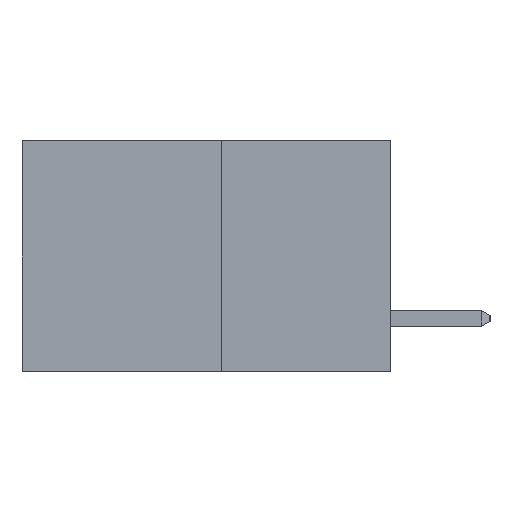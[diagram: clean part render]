
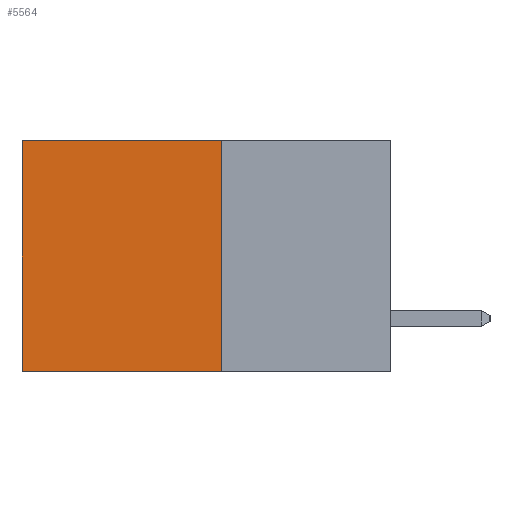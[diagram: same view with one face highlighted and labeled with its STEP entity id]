
A CAD part, left-side view. The second image highlights one B-rep face of the part: STEP entity #5564.
In plain terms, the highlighted planar face has unit normal (-1, 0, 0).
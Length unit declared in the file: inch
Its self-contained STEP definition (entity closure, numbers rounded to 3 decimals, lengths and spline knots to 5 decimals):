
#116 = VERTEX_POINT ( 'NONE', #3223 ) ;
#127 = EDGE_CURVE ( 'NONE', #1532, #116, #7901, .T. ) ;
#175 = ORIENTED_EDGE ( 'NONE', *, *, #199, .T. ) ;
#199 = EDGE_CURVE ( 'NONE', #2654, #116, #7151, .T. ) ;
#217 = VECTOR ( 'NONE', #4438, 39.37008 ) ;
#226 = ORIENTED_EDGE ( 'NONE', *, *, #127, .F. ) ;
#299 = DIRECTION ( 'NONE',  ( 0., 1., 0. ) ) ;
#313 = ORIENTED_EDGE ( 'NONE', *, *, #3070, .F. ) ;
#405 = ORIENTED_EDGE ( 'NONE', *, *, #1377, .T. ) ;
#804 = DIRECTION ( 'NONE',  ( 0., 1., 0. ) ) ;
#1377 = EDGE_CURVE ( 'NONE', #5748, #2654, #5224, .T. ) ;
#1532 = VERTEX_POINT ( 'NONE', #8156 ) ;
#1837 = FACE_OUTER_BOUND ( 'NONE', #6592, .T. ) ;
#2405 = CARTESIAN_POINT ( 'NONE',  ( 0.277, 0.27, -0.37 ) ) ;
#2654 = VERTEX_POINT ( 'NONE', #3003 ) ;
#2726 = VECTOR ( 'NONE', #6713, 39.37008 ) ;
#3003 = CARTESIAN_POINT ( 'NONE',  ( 0.277, 0.59, 0. ) ) ;
#3070 = EDGE_CURVE ( 'NONE', #5748, #1532, #3132, .T. ) ;
#3132 = LINE ( 'NONE', #2405, #2726 ) ;
#3180 = CARTESIAN_POINT ( 'NONE',  ( 0.277, 0.59, -0.37 ) ) ;
#3223 = CARTESIAN_POINT ( 'NONE',  ( 0.277, 0.59, -0.37 ) ) ;
#3611 = DIRECTION ( 'NONE',  ( 1., 0., 0. ) ) ;
#3656 = DIRECTION ( 'NONE',  ( 0., 0., -1. ) ) ;
#3870 = CARTESIAN_POINT ( 'NONE',  ( 0.277, 0.27, -0.37 ) ) ;
#4122 = PLANE ( 'NONE',  #4773 ) ;
#4438 = DIRECTION ( 'NONE',  ( 0., 0., -1. ) ) ;
#4773 = AXIS2_PLACEMENT_3D ( 'NONE', #3870, #3611, #3656 ) ;
#5224 = LINE ( 'NONE', #6481, #8258 ) ;
#5564 = ADVANCED_FACE ( 'NONE', ( #1837 ), #4122, .F. ) ;
#5680 = CARTESIAN_POINT ( 'NONE',  ( 0.277, 0.27, -0.37 ) ) ;
#5748 = VERTEX_POINT ( 'NONE', #8255 ) ;
#6481 = CARTESIAN_POINT ( 'NONE',  ( 0.277, 0.27, 0. ) ) ;
#6592 = EDGE_LOOP ( 'NONE', ( #175, #226, #313, #405 ) ) ;
#6713 = DIRECTION ( 'NONE',  ( 0., 0., -1. ) ) ;
#7151 = LINE ( 'NONE', #3180, #217 ) ;
#7717 = VECTOR ( 'NONE', #804, 39.37008 ) ;
#7901 = LINE ( 'NONE', #5680, #7717 ) ;
#8156 = CARTESIAN_POINT ( 'NONE',  ( 0.277, 0.27, -0.37 ) ) ;
#8255 = CARTESIAN_POINT ( 'NONE',  ( 0.277, 0.27, 0. ) ) ;
#8258 = VECTOR ( 'NONE', #299, 39.37008 ) ;
